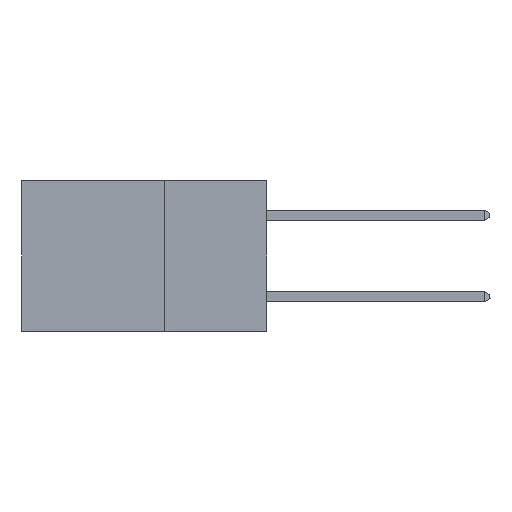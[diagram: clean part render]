
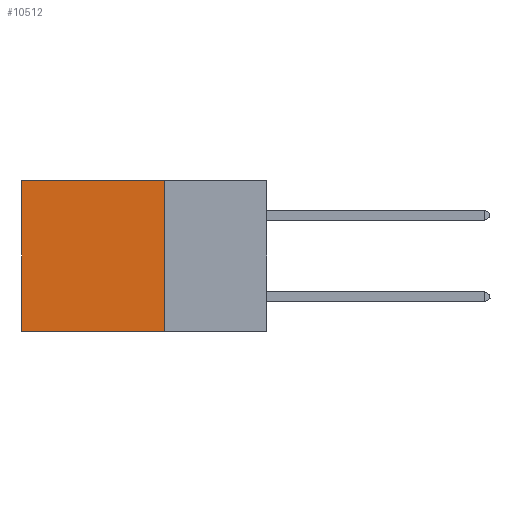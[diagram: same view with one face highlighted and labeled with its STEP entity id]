
A CAD part, left-side view. The second image highlights one B-rep face of the part: STEP entity #10512.
In plain terms, the highlighted planar face has unit normal (-1, 0, 0).
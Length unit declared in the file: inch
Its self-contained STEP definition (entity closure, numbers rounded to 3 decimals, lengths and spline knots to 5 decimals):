
#607 = CARTESIAN_POINT ( 'NONE',  ( 0.2875, 0.6, -0.37 ) ) ;
#631 = DIRECTION ( 'NONE',  ( 0., 0., -1. ) ) ;
#1052 = PLANE ( 'NONE',  #8868 ) ;
#1094 = ORIENTED_EDGE ( 'NONE', *, *, #20380, .T. ) ;
#1152 = CARTESIAN_POINT ( 'NONE',  ( 0.2875, 0.25, -0.37 ) ) ;
#1448 = CARTESIAN_POINT ( 'NONE',  ( 0.2875, 0.25, -0.37 ) ) ;
#1940 = ORIENTED_EDGE ( 'NONE', *, *, #17415, .F. ) ;
#2264 = CARTESIAN_POINT ( 'NONE',  ( 0.2875, 0.6, 0. ) ) ;
#3647 = LINE ( 'NONE', #8991, #15149 ) ;
#4077 = EDGE_CURVE ( 'NONE', #11231, #7132, #7151, .T. ) ;
#4626 = VECTOR ( 'NONE', #7460, 39.37008 ) ;
#7132 = VERTEX_POINT ( 'NONE', #15560 ) ;
#7151 = LINE ( 'NONE', #21841, #4626 ) ;
#7211 = DIRECTION ( 'NONE',  ( 0., 0., -1. ) ) ;
#7310 = ORIENTED_EDGE ( 'NONE', *, *, #4077, .T. ) ;
#7460 = DIRECTION ( 'NONE',  ( 0., 1., 0. ) ) ;
#8296 = DIRECTION ( 'NONE',  ( 1., 0., 0. ) ) ;
#8868 = AXIS2_PLACEMENT_3D ( 'NONE', #13586, #8296, #9729 ) ;
#8991 = CARTESIAN_POINT ( 'NONE',  ( 0.2875, 0.25, 0. ) ) ;
#9623 = CARTESIAN_POINT ( 'NONE',  ( 0.2875, 0.25, 0. ) ) ;
#9729 = DIRECTION ( 'NONE',  ( 0., 0., -1. ) ) ;
#9890 = LINE ( 'NONE', #2264, #20219 ) ;
#10512 = ADVANCED_FACE ( 'NONE', ( #16392 ), #1052, .F. ) ;
#11231 = VERTEX_POINT ( 'NONE', #9623 ) ;
#12699 = VERTEX_POINT ( 'NONE', #607 ) ;
#13586 = CARTESIAN_POINT ( 'NONE',  ( 0.2875, 0.25, 0. ) ) ;
#13855 = LINE ( 'NONE', #1152, #14981 ) ;
#13980 = ORIENTED_EDGE ( 'NONE', *, *, #18490, .F. ) ;
#14981 = VECTOR ( 'NONE', #23067, 39.37008 ) ;
#15149 = VECTOR ( 'NONE', #7211, 39.37008 ) ;
#15560 = CARTESIAN_POINT ( 'NONE',  ( 0.2875, 0.6, 0. ) ) ;
#16392 = FACE_OUTER_BOUND ( 'NONE', #17195, .T. ) ;
#17195 = EDGE_LOOP ( 'NONE', ( #1094, #13980, #1940, #7310 ) ) ;
#17415 = EDGE_CURVE ( 'NONE', #11231, #19711, #3647, .T. ) ;
#18490 = EDGE_CURVE ( 'NONE', #19711, #12699, #13855, .T. ) ;
#19711 = VERTEX_POINT ( 'NONE', #1448 ) ;
#20219 = VECTOR ( 'NONE', #631, 39.37008 ) ;
#20380 = EDGE_CURVE ( 'NONE', #7132, #12699, #9890, .T. ) ;
#21841 = CARTESIAN_POINT ( 'NONE',  ( 0.2875, 0.25, 0. ) ) ;
#23067 = DIRECTION ( 'NONE',  ( 0., 1., 0. ) ) ;
